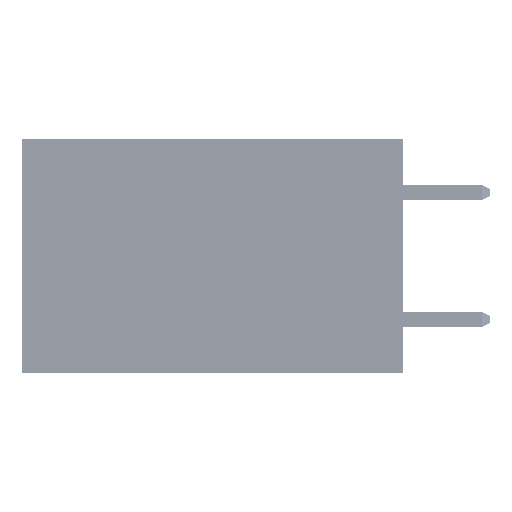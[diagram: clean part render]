
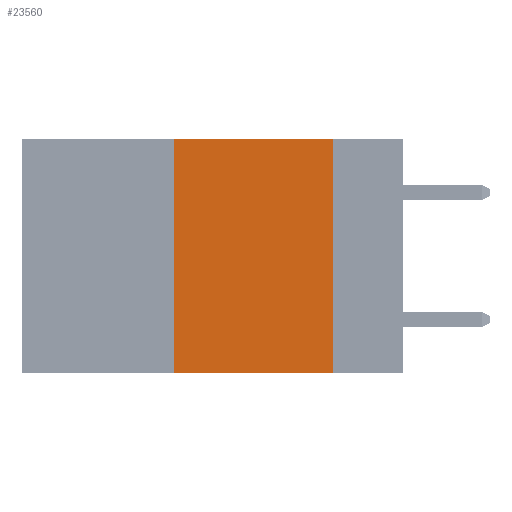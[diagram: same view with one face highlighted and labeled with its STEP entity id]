
A CAD part, left-side view. The second image highlights one B-rep face of the part: STEP entity #23560.
In plain terms, the highlighted planar face has unit normal (-1, 0, 0).
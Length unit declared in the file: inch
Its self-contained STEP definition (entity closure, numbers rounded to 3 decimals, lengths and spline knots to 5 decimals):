
#2018 = DIRECTION ( 'NONE',  ( 0., -1., 0. ) ) ;
#2361 = VECTOR ( 'NONE', #2018, 39.37008 ) ;
#2537 = CARTESIAN_POINT ( 'NONE',  ( 0., 0.6, -0.37 ) ) ;
#3920 = PLANE ( 'NONE',  #49435 ) ;
#4481 = CARTESIAN_POINT ( 'NONE',  ( 0., 0.36, 0. ) ) ;
#7286 = CARTESIAN_POINT ( 'NONE',  ( 0., 0.6, 0. ) ) ;
#8123 = CARTESIAN_POINT ( 'NONE',  ( 0., 0.36, -0.37 ) ) ;
#9663 = LINE ( 'NONE', #50267, #38186 ) ;
#9752 = EDGE_LOOP ( 'NONE', ( #49861, #40451, #50722, #43783 ) ) ;
#9990 = EDGE_CURVE ( 'NONE', #17201, #18949, #48913, .T. ) ;
#15427 = VERTEX_POINT ( 'NONE', #8123 ) ;
#17201 = VERTEX_POINT ( 'NONE', #35197 ) ;
#18047 = CARTESIAN_POINT ( 'NONE',  ( 0., 0.6, 0. ) ) ;
#18724 = EDGE_CURVE ( 'NONE', #25975, #17201, #45067, .T. ) ;
#18949 = VERTEX_POINT ( 'NONE', #35913 ) ;
#19094 = VECTOR ( 'NONE', #39303, 39.37008 ) ;
#23268 = LINE ( 'NONE', #2537, #2361 ) ;
#23487 = VECTOR ( 'NONE', #50325, 39.37008 ) ;
#23560 = ADVANCED_FACE ( 'NONE', ( #40581 ), #3920, .F. ) ;
#24990 = DIRECTION ( 'NONE',  ( 0., 0., -1. ) ) ;
#25975 = VERTEX_POINT ( 'NONE', #4481 ) ;
#29392 = EDGE_CURVE ( 'NONE', #15427, #25975, #9663, .T. ) ;
#35197 = CARTESIAN_POINT ( 'NONE',  ( 0., 0.11, 0. ) ) ;
#35913 = CARTESIAN_POINT ( 'NONE',  ( 0., 0.11, -0.37 ) ) ;
#37814 = DIRECTION ( 'NONE',  ( 0., 0., 1. ) ) ;
#38186 = VECTOR ( 'NONE', #37814, 39.37008 ) ;
#39303 = DIRECTION ( 'NONE',  ( 0., 0., -1. ) ) ;
#40250 = EDGE_CURVE ( 'NONE', #15427, #18949, #23268, .T. ) ;
#40451 = ORIENTED_EDGE ( 'NONE', *, *, #18724, .F. ) ;
#40581 = FACE_OUTER_BOUND ( 'NONE', #9752, .T. ) ;
#43783 = ORIENTED_EDGE ( 'NONE', *, *, #40250, .T. ) ;
#45067 = LINE ( 'NONE', #18047, #23487 ) ;
#45209 = DIRECTION ( 'NONE',  ( 1., 0., 0. ) ) ;
#48913 = LINE ( 'NONE', #51239, #19094 ) ;
#49435 = AXIS2_PLACEMENT_3D ( 'NONE', #7286, #45209, #24990 ) ;
#49861 = ORIENTED_EDGE ( 'NONE', *, *, #9990, .F. ) ;
#50267 = CARTESIAN_POINT ( 'NONE',  ( 0., 0.36, 0. ) ) ;
#50325 = DIRECTION ( 'NONE',  ( 0., -1., 0. ) ) ;
#50722 = ORIENTED_EDGE ( 'NONE', *, *, #29392, .F. ) ;
#51239 = CARTESIAN_POINT ( 'NONE',  ( 0., 0.11, 0. ) ) ;
